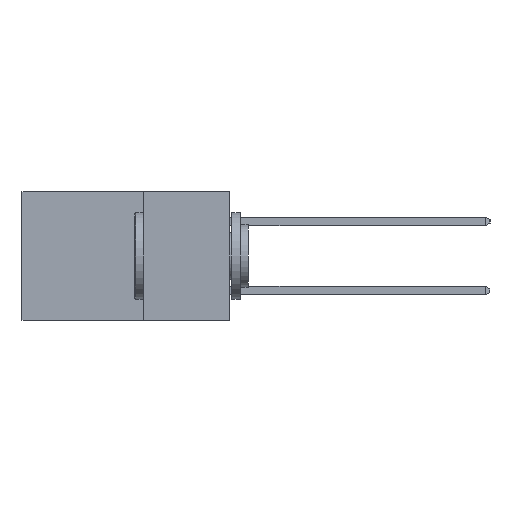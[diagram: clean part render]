
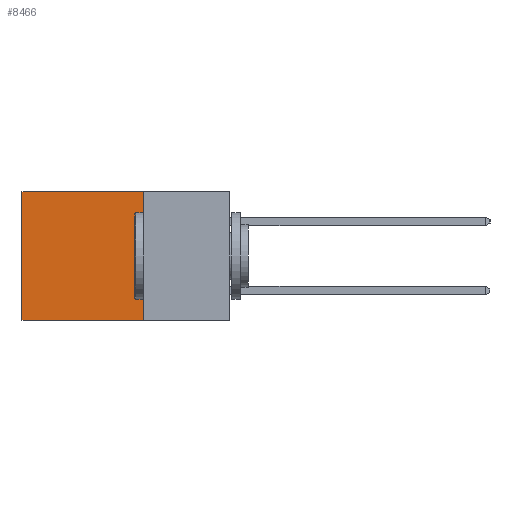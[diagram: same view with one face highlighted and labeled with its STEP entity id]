
A CAD part, left-side view. The second image highlights one B-rep face of the part: STEP entity #8466.
In plain terms, the highlighted planar face has unit normal (-1, 0, 0).
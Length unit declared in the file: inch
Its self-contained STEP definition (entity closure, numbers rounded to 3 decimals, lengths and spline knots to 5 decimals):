
#5 = ORIENTED_EDGE ( 'NONE', *, *, #9157, .F. ) ;
#280 = ORIENTED_EDGE ( 'NONE', *, *, #7862, .F. ) ;
#457 = DIRECTION ( 'NONE',  ( 0., 1., 0. ) ) ;
#500 = CARTESIAN_POINT ( 'NONE',  ( 0.298, 0.25, 0. ) ) ;
#806 = EDGE_CURVE ( 'NONE', #6280, #1266, #2838, .T. ) ;
#813 = CARTESIAN_POINT ( 'NONE',  ( 0.298, 0.25, 0. ) ) ;
#1186 = VERTEX_POINT ( 'NONE', #813 ) ;
#1266 = VERTEX_POINT ( 'NONE', #8511 ) ;
#1449 = DIRECTION ( 'NONE',  ( 1., 0., 0. ) ) ;
#1514 = VECTOR ( 'NONE', #4036, 39.37008 ) ;
#1551 = LINE ( 'NONE', #4170, #5968 ) ;
#1813 = VERTEX_POINT ( 'NONE', #6562 ) ;
#2697 = ORIENTED_EDGE ( 'NONE', *, *, #8456, .T. ) ;
#2838 = LINE ( 'NONE', #7628, #9699 ) ;
#3175 = CARTESIAN_POINT ( 'NONE',  ( 0.298, 0.25, -0.37 ) ) ;
#3293 = DIRECTION ( 'NONE',  ( 0., 0., -1. ) ) ;
#3840 = LINE ( 'NONE', #3175, #1514 ) ;
#4036 = DIRECTION ( 'NONE',  ( 0., 1., 0. ) ) ;
#4170 = CARTESIAN_POINT ( 'NONE',  ( 0.298, 0.25, 0. ) ) ;
#4825 = LINE ( 'NONE', #6759, #7276 ) ;
#5853 = PLANE ( 'NONE',  #6978 ) ;
#5968 = VECTOR ( 'NONE', #3293, 39.37008 ) ;
#6280 = VERTEX_POINT ( 'NONE', #6398 ) ;
#6398 = CARTESIAN_POINT ( 'NONE',  ( 0.298, 0.6, 0. ) ) ;
#6405 = DIRECTION ( 'NONE',  ( 0., 0., -1. ) ) ;
#6562 = CARTESIAN_POINT ( 'NONE',  ( 0.298, 0.25, -0.37 ) ) ;
#6608 = ORIENTED_EDGE ( 'NONE', *, *, #806, .T. ) ;
#6619 = EDGE_LOOP ( 'NONE', ( #6608, #5, #280, #2697 ) ) ;
#6759 = CARTESIAN_POINT ( 'NONE',  ( 0.298, 0.25, 0. ) ) ;
#6978 = AXIS2_PLACEMENT_3D ( 'NONE', #500, #1449, #7683 ) ;
#7276 = VECTOR ( 'NONE', #457, 39.37008 ) ;
#7628 = CARTESIAN_POINT ( 'NONE',  ( 0.298, 0.6, 0. ) ) ;
#7683 = DIRECTION ( 'NONE',  ( 0., 0., -1. ) ) ;
#7862 = EDGE_CURVE ( 'NONE', #1186, #1813, #1551, .T. ) ;
#8456 = EDGE_CURVE ( 'NONE', #1186, #6280, #4825, .T. ) ;
#8466 = ADVANCED_FACE ( 'NONE', ( #9174 ), #5853, .F. ) ;
#8511 = CARTESIAN_POINT ( 'NONE',  ( 0.298, 0.6, -0.37 ) ) ;
#9157 = EDGE_CURVE ( 'NONE', #1813, #1266, #3840, .T. ) ;
#9174 = FACE_OUTER_BOUND ( 'NONE', #6619, .T. ) ;
#9699 = VECTOR ( 'NONE', #6405, 39.37008 ) ;
